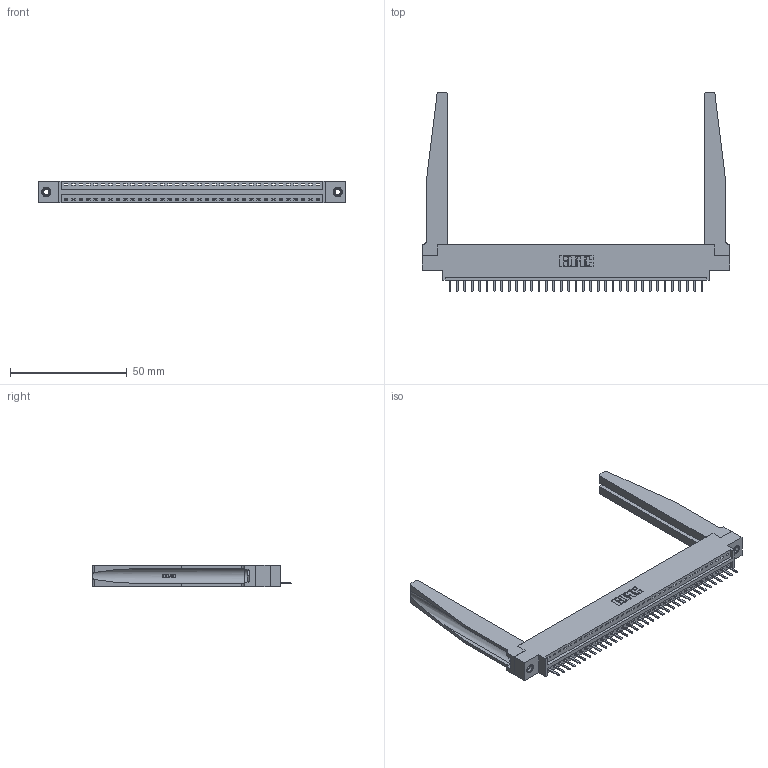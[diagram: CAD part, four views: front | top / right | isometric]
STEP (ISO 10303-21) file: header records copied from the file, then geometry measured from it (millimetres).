
FILE_DESCRIPTION (( 'STEP AP203' ), '1' );
FILE_NAME ('346-035-520-678.STEP', '2022-05-06T22:37:48', ( '' ), ( '' ), 'SwSTEP 2.0', 'SolidWorks 2020', '' );
FILE_SCHEMA (( 'CONFIG_CONTROL_DESIGN' ));
Length unit declared in the file: inch
Products named in the file (5): 346-035-520-678; 345-292-001_345-293-120; 345-250-001_345-250-001-102; 346-220-078_345-220-078; 346 Part_0.170 Offset - 0.156 Dia-TH
Assembly tree (40 placements, depth 2):
  346-035-520-678
    346 Part_0.170 Offset - 0.156 Dia-TH
    345-292-001_345-293-120  x35
    346-220-078_345-220-078  x2
    345-250-001_345-250-001-102  x2
Bounding box: 131.7 x 85.29 x 9.4 mm (x, y, z)
Volume: 19193.8 mm3; surface area: 21675.6 mm2
Topology: 40 solids, 40 shells, 2544 faces, 7425 edges, 4846 vertices
Faces by surface type: plane 1706, cylinder 786, bspline 36, cone 12, torus 4
Entity records: 28074 total; most frequent: CARTESIAN_POINT 5742, ORIENTED_EDGE 4586, DIRECTION 4045, EDGE_CURVE 2293, LINE 1923, VECTOR 1923, VERTEX_POINT 1520, AXIS2_PLACEMENT_3D 1061
